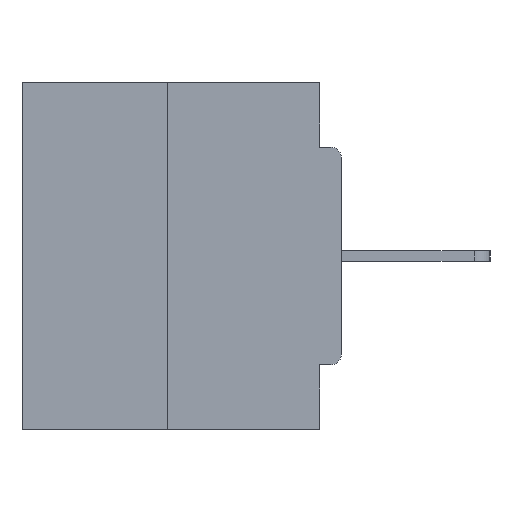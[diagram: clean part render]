
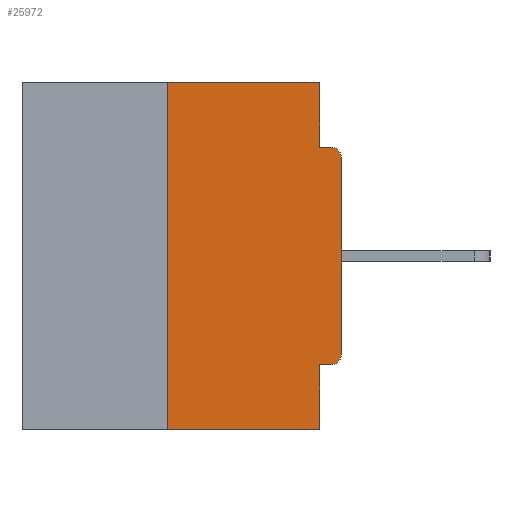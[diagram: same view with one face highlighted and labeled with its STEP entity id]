
A CAD part, left-side view. The second image highlights one B-rep face of the part: STEP entity #25972.
In plain terms, the highlighted planar face has unit normal (-1, 0, 0).
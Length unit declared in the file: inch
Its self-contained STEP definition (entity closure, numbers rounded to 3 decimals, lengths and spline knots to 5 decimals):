
#616 = ORIENTED_EDGE ( 'NONE', *, *, #15033, .T. ) ;
#701 = DIRECTION ( 'NONE',  ( 0., -1., 0. ) ) ;
#814 = ORIENTED_EDGE ( 'NONE', *, *, #32633, .F. ) ;
#1522 = DIRECTION ( 'NONE',  ( 0., 0., -1. ) ) ;
#1581 = VECTOR ( 'NONE', #3717, 39.37008 ) ;
#1726 = EDGE_CURVE ( 'NONE', #1762, #14378, #6555, .T. ) ;
#1762 = VERTEX_POINT ( 'NONE', #8029 ) ;
#2020 = DIRECTION ( 'NONE',  ( 0., 0., 1. ) ) ;
#2306 = CARTESIAN_POINT ( 'NONE',  ( 0., 0.25, 0. ) ) ;
#2341 = ORIENTED_EDGE ( 'NONE', *, *, #1726, .T. ) ;
#2707 = DIRECTION ( 'NONE',  ( -1., 0., 0. ) ) ;
#2934 = VECTOR ( 'NONE', #27157, 39.37008 ) ;
#3602 = VECTOR ( 'NONE', #17806, 39.37008 ) ;
#3717 = DIRECTION ( 'NONE',  ( 0., -1., 0. ) ) ;
#4084 = VERTEX_POINT ( 'NONE', #22527 ) ;
#4854 = ORIENTED_EDGE ( 'NONE', *, *, #16550, .F. ) ;
#5539 = VERTEX_POINT ( 'NONE', #2306 ) ;
#5585 = VERTEX_POINT ( 'NONE', #14859 ) ;
#5839 = VERTEX_POINT ( 'NONE', #16658 ) ;
#6169 = CARTESIAN_POINT ( 'NONE',  ( 0., 0.015, -0.1085 ) ) ;
#6411 = EDGE_CURVE ( 'NONE', #5539, #4084, #29159, .T. ) ;
#6555 = CIRCLE ( 'NONE', #30125, 0.015 ) ;
#7159 = LINE ( 'NONE', #29797, #10546 ) ;
#7486 = VECTOR ( 'NONE', #29480, 39.37008 ) ;
#7736 = ORIENTED_EDGE ( 'NONE', *, *, #25707, .T. ) ;
#8029 = CARTESIAN_POINT ( 'NONE',  ( 0., 0.015, -0.4065 ) ) ;
#9142 = DIRECTION ( 'NONE',  ( 0., 0., -1. ) ) ;
#9635 = DIRECTION ( 'NONE',  ( 1., 0., 0. ) ) ;
#10546 = VECTOR ( 'NONE', #2020, 39.37008 ) ;
#10707 = LINE ( 'NONE', #25968, #16016 ) ;
#11224 = ORIENTED_EDGE ( 'NONE', *, *, #21798, .F. ) ;
#11561 = CARTESIAN_POINT ( 'NONE',  ( 0., 0.031, -0.5 ) ) ;
#12263 = EDGE_CURVE ( 'NONE', #5839, #5585, #31319, .T. ) ;
#13431 = DIRECTION ( 'NONE',  ( 0., -1., 0. ) ) ;
#14378 = VERTEX_POINT ( 'NONE', #24382 ) ;
#14427 = ORIENTED_EDGE ( 'NONE', *, *, #16904, .T. ) ;
#14844 = PLANE ( 'NONE',  #31422 ) ;
#14859 = CARTESIAN_POINT ( 'NONE',  ( 0., 0.015, -0.0935 ) ) ;
#15033 = EDGE_CURVE ( 'NONE', #17083, #15229, #16099, .T. ) ;
#15229 = VERTEX_POINT ( 'NONE', #11561 ) ;
#15602 = CARTESIAN_POINT ( 'NONE',  ( 0., 0.46, -0.5 ) ) ;
#16016 = VECTOR ( 'NONE', #28473, 39.37008 ) ;
#16099 = LINE ( 'NONE', #15602, #17809 ) ;
#16550 = EDGE_CURVE ( 'NONE', #20226, #15229, #21819, .T. ) ;
#16658 = CARTESIAN_POINT ( 'NONE',  ( 0., 0.031, -0.0935 ) ) ;
#16904 = EDGE_CURVE ( 'NONE', #30138, #5585, #32904, .T. ) ;
#17083 = VERTEX_POINT ( 'NONE', #22442 ) ;
#17114 = CARTESIAN_POINT ( 'NONE',  ( 0., 0.031, -0.5 ) ) ;
#17806 = DIRECTION ( 'NONE',  ( 0., 0., 1. ) ) ;
#17809 = VECTOR ( 'NONE', #13431, 39.37008 ) ;
#18307 = EDGE_LOOP ( 'NONE', ( #19706, #11224, #616, #4854, #30523, #2341, #7736, #14427, #24356, #814 ) ) ;
#18438 = AXIS2_PLACEMENT_3D ( 'NONE', #6169, #21448, #1522 ) ;
#19250 = LINE ( 'NONE', #21972, #7486 ) ;
#19706 = ORIENTED_EDGE ( 'NONE', *, *, #6411, .F. ) ;
#19852 = CARTESIAN_POINT ( 'NONE',  ( 0., 0.46, 0. ) ) ;
#20226 = VERTEX_POINT ( 'NONE', #30925 ) ;
#21448 = DIRECTION ( 'NONE',  ( -1., 0., 0. ) ) ;
#21798 = EDGE_CURVE ( 'NONE', #17083, #5539, #7159, .T. ) ;
#21819 = LINE ( 'NONE', #17114, #2934 ) ;
#21972 = CARTESIAN_POINT ( 'NONE',  ( 0., 0., -0.4065 ) ) ;
#22442 = CARTESIAN_POINT ( 'NONE',  ( 0., 0.25, -0.5 ) ) ;
#22527 = CARTESIAN_POINT ( 'NONE',  ( 0., 0.031, 0. ) ) ;
#23131 = DIRECTION ( 'NONE',  ( 0., 0., -1. ) ) ;
#23144 = CARTESIAN_POINT ( 'NONE',  ( 0., 0., -0.0935 ) ) ;
#23326 = CARTESIAN_POINT ( 'NONE',  ( 0., 0., 0. ) ) ;
#24356 = ORIENTED_EDGE ( 'NONE', *, *, #12263, .F. ) ;
#24382 = CARTESIAN_POINT ( 'NONE',  ( 0., 0., -0.3915 ) ) ;
#25643 = CARTESIAN_POINT ( 'NONE',  ( 0., 0.015, -0.3915 ) ) ;
#25707 = EDGE_CURVE ( 'NONE', #14378, #30138, #25999, .T. ) ;
#25968 = CARTESIAN_POINT ( 'NONE',  ( 0., 0.031, 0. ) ) ;
#25972 = ADVANCED_FACE ( 'NONE', ( #32424 ), #14844, .F. ) ;
#25999 = LINE ( 'NONE', #23326, #3602 ) ;
#27157 = DIRECTION ( 'NONE',  ( 0., 0., -1. ) ) ;
#28142 = CARTESIAN_POINT ( 'NONE',  ( 0., 0., -0.1085 ) ) ;
#28473 = DIRECTION ( 'NONE',  ( 0., 0., -1. ) ) ;
#29159 = LINE ( 'NONE', #32014, #1581 ) ;
#29480 = DIRECTION ( 'NONE',  ( 0., 1., 0. ) ) ;
#29797 = CARTESIAN_POINT ( 'NONE',  ( 0., 0.25, 0. ) ) ;
#30125 = AXIS2_PLACEMENT_3D ( 'NONE', #25643, #2707, #23131 ) ;
#30138 = VERTEX_POINT ( 'NONE', #28142 ) ;
#30523 = ORIENTED_EDGE ( 'NONE', *, *, #32817, .F. ) ;
#30925 = CARTESIAN_POINT ( 'NONE',  ( 0., 0.031, -0.4065 ) ) ;
#31319 = LINE ( 'NONE', #23144, #31417 ) ;
#31417 = VECTOR ( 'NONE', #701, 39.37008 ) ;
#31422 = AXIS2_PLACEMENT_3D ( 'NONE', #19852, #9635, #9142 ) ;
#32014 = CARTESIAN_POINT ( 'NONE',  ( 0., 0.46, 0. ) ) ;
#32424 = FACE_OUTER_BOUND ( 'NONE', #18307, .T. ) ;
#32633 = EDGE_CURVE ( 'NONE', #4084, #5839, #10707, .T. ) ;
#32817 = EDGE_CURVE ( 'NONE', #1762, #20226, #19250, .T. ) ;
#32904 = CIRCLE ( 'NONE', #18438, 0.015 ) ;
